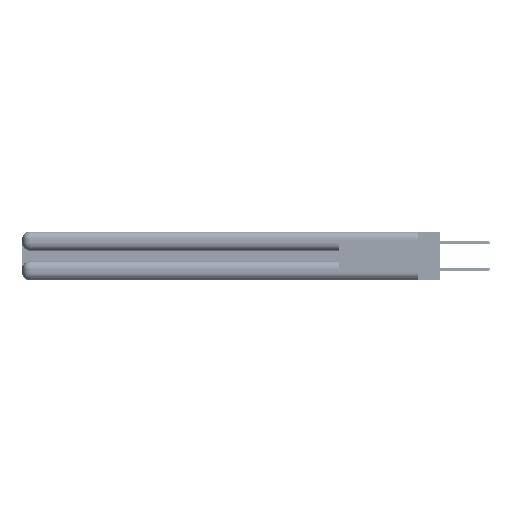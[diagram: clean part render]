
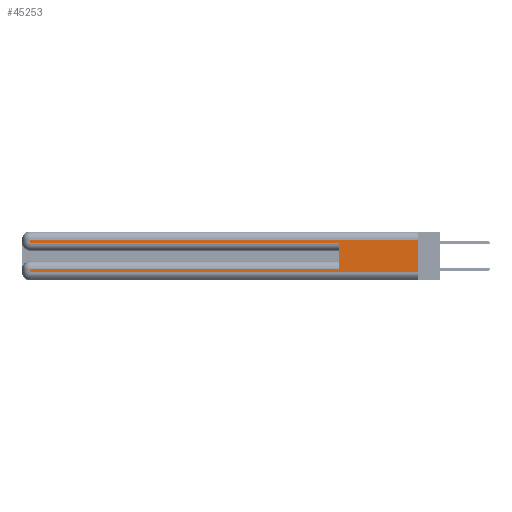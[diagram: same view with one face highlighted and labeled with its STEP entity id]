
A CAD part, left-side view. The second image highlights one B-rep face of the part: STEP entity #45253.
In plain terms, the highlighted planar face has unit normal (-1, 0, 0).
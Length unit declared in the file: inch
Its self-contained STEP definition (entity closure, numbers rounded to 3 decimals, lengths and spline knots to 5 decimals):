
#804 = LINE ( 'NONE', #31254, #15939 ) ;
#1005 = EDGE_CURVE ( 'NONE', #45553, #36986, #32992, .T. ) ;
#1194 = CARTESIAN_POINT ( 'NONE',  ( 0., 2.94, 0.37 ) ) ;
#1388 = LINE ( 'NONE', #26170, #43557 ) ;
#1970 = CARTESIAN_POINT ( 'NONE',  ( 0., 0.6, 0.285 ) ) ;
#3256 = CARTESIAN_POINT ( 'NONE',  ( 0., 0.6, 0.085 ) ) ;
#5655 = DIRECTION ( 'NONE',  ( 0., 0., -1. ) ) ;
#6533 = CARTESIAN_POINT ( 'NONE',  ( 0., 0.6, 0.145 ) ) ;
#7339 = CARTESIAN_POINT ( 'NONE',  ( 0., 2.94, 0.31 ) ) ;
#7798 = VECTOR ( 'NONE', #27204, 39.37008 ) ;
#8345 = VERTEX_POINT ( 'NONE', #54192 ) ;
#10921 = DIRECTION ( 'NONE',  ( 0., 0., 1. ) ) ;
#11546 = LINE ( 'NONE', #1194, #37810 ) ;
#12640 = VECTOR ( 'NONE', #26079, 39.37008 ) ;
#12670 = ORIENTED_EDGE ( 'NONE', *, *, #1005, .T. ) ;
#14018 = LINE ( 'NONE', #49060, #12640 ) ;
#15217 = VERTEX_POINT ( 'NONE', #40167 ) ;
#15615 = VERTEX_POINT ( 'NONE', #1970 ) ;
#15939 = VECTOR ( 'NONE', #53854, 39.37008 ) ;
#18142 = CARTESIAN_POINT ( 'NONE',  ( 0., 2.94, 0.37 ) ) ;
#18339 = EDGE_CURVE ( 'NONE', #46742, #38222, #14018, .T. ) ;
#18890 = CARTESIAN_POINT ( 'NONE',  ( 0., 0., 0.37 ) ) ;
#19941 = VECTOR ( 'NONE', #10921, 39.37008 ) ;
#20269 = AXIS2_PLACEMENT_3D ( 'NONE', #18890, #28152, #36483 ) ;
#21560 = ORIENTED_EDGE ( 'NONE', *, *, #36475, .F. ) ;
#22570 = CARTESIAN_POINT ( 'NONE',  ( 0., 2.94, 0.06 ) ) ;
#22575 = VECTOR ( 'NONE', #48847, 39.37008 ) ;
#25350 = LINE ( 'NONE', #31243, #22575 ) ;
#25438 = ORIENTED_EDGE ( 'NONE', *, *, #43423, .T. ) ;
#26079 = DIRECTION ( 'NONE',  ( 0., 1., 0. ) ) ;
#26170 = CARTESIAN_POINT ( 'NONE',  ( 0., 0., 0.285 ) ) ;
#26656 = CARTESIAN_POINT ( 'NONE',  ( 0., 0., 0.31 ) ) ;
#27204 = DIRECTION ( 'NONE',  ( 0., 0., -1. ) ) ;
#28022 = ORIENTED_EDGE ( 'NONE', *, *, #34105, .T. ) ;
#28152 = DIRECTION ( 'NONE',  ( 1., 0., 0. ) ) ;
#30953 = VECTOR ( 'NONE', #38686, 39.37008 ) ;
#31243 = CARTESIAN_POINT ( 'NONE',  ( 0., 0., 0.37 ) ) ;
#31254 = CARTESIAN_POINT ( 'NONE',  ( 0., 0., 0.06 ) ) ;
#31693 = LINE ( 'NONE', #6533, #19941 ) ;
#32992 = LINE ( 'NONE', #56253, #30953 ) ;
#34105 = EDGE_CURVE ( 'NONE', #15217, #15615, #1388, .T. ) ;
#34494 = ORIENTED_EDGE ( 'NONE', *, *, #55059, .F. ) ;
#36475 = EDGE_CURVE ( 'NONE', #45553, #8345, #25350, .T. ) ;
#36483 = DIRECTION ( 'NONE',  ( 0., 0., -1. ) ) ;
#36986 = VERTEX_POINT ( 'NONE', #7339 ) ;
#37118 = ORIENTED_EDGE ( 'NONE', *, *, #56061, .T. ) ;
#37229 = PLANE ( 'NONE',  #20269 ) ;
#37810 = VECTOR ( 'NONE', #5655, 39.37008 ) ;
#37938 = ORIENTED_EDGE ( 'NONE', *, *, #18339, .T. ) ;
#38222 = VERTEX_POINT ( 'NONE', #47527 ) ;
#38502 = EDGE_CURVE ( 'NONE', #40024, #8345, #804, .T. ) ;
#38686 = DIRECTION ( 'NONE',  ( 0., 1., 0. ) ) ;
#40024 = VERTEX_POINT ( 'NONE', #22570 ) ;
#40167 = CARTESIAN_POINT ( 'NONE',  ( 0., 2.94, 0.285 ) ) ;
#41644 = LINE ( 'NONE', #18142, #7798 ) ;
#43423 = EDGE_CURVE ( 'NONE', #38222, #40024, #41644, .T. ) ;
#43557 = VECTOR ( 'NONE', #48205, 39.37008 ) ;
#44454 = EDGE_LOOP ( 'NONE', ( #21560, #12670, #37118, #28022, #34494, #37938, #25438, #54008 ) ) ;
#45253 = ADVANCED_FACE ( 'NONE', ( #55973 ), #37229, .F. ) ;
#45553 = VERTEX_POINT ( 'NONE', #26656 ) ;
#46742 = VERTEX_POINT ( 'NONE', #3256 ) ;
#47527 = CARTESIAN_POINT ( 'NONE',  ( 0., 2.94, 0.085 ) ) ;
#48205 = DIRECTION ( 'NONE',  ( 0., -1., 0. ) ) ;
#48847 = DIRECTION ( 'NONE',  ( 0., 0., -1. ) ) ;
#49060 = CARTESIAN_POINT ( 'NONE',  ( 0., 0., 0.085 ) ) ;
#53854 = DIRECTION ( 'NONE',  ( 0., -1., 0. ) ) ;
#54008 = ORIENTED_EDGE ( 'NONE', *, *, #38502, .T. ) ;
#54192 = CARTESIAN_POINT ( 'NONE',  ( 0., 0., 0.06 ) ) ;
#55059 = EDGE_CURVE ( 'NONE', #46742, #15615, #31693, .T. ) ;
#55973 = FACE_OUTER_BOUND ( 'NONE', #44454, .T. ) ;
#56061 = EDGE_CURVE ( 'NONE', #36986, #15217, #11546, .T. ) ;
#56253 = CARTESIAN_POINT ( 'NONE',  ( 0., 0., 0.31 ) ) ;
